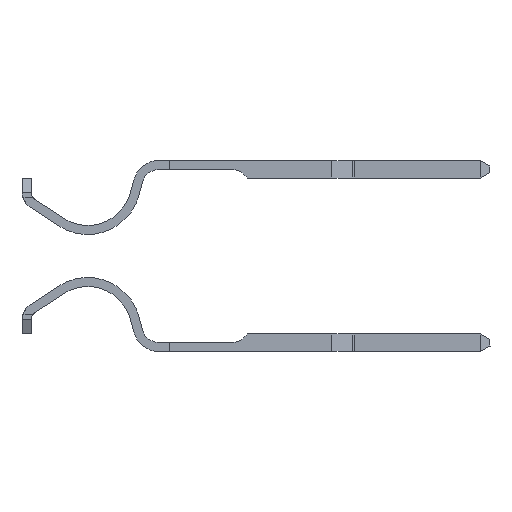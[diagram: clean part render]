
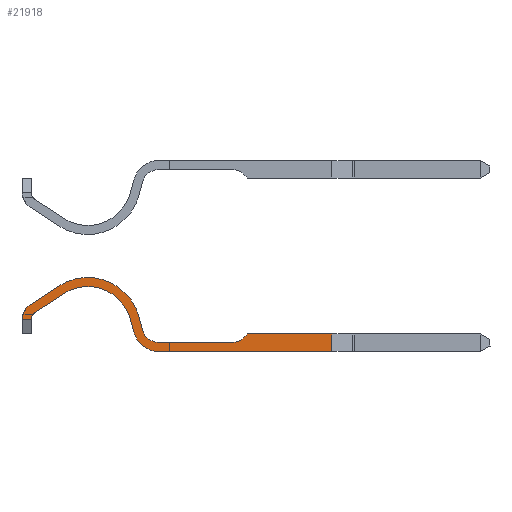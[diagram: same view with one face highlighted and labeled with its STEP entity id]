
A CAD part, left-side view. The second image highlights one B-rep face of the part: STEP entity #21918.
In plain terms, the highlighted face is planar.
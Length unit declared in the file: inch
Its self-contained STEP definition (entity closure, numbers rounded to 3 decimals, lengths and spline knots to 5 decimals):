
#345 = DIRECTION ( 'NONE',  ( 0., 0., -1. ) ) ;
#789 = DIRECTION ( 'NONE',  ( 0.836, 0.549, 0. ) ) ;
#810 = DIRECTION ( 'NONE',  ( 1., 0., 0. ) ) ;
#1173 = CARTESIAN_POINT ( 'NONE',  ( 0.43721, 0.04723, 0.025 ) ) ;
#1395 = DIRECTION ( 'NONE',  ( 1., 0., 0. ) ) ;
#1508 = VERTEX_POINT ( 'NONE', #23892 ) ;
#1675 = CARTESIAN_POINT ( 'NONE',  ( 0.18604, 0.10646, 0.025 ) ) ;
#1725 = VERTEX_POINT ( 'NONE', #7001 ) ;
#1872 = ORIENTED_EDGE ( 'NONE', *, *, #14459, .T. ) ;
#1982 = EDGE_CURVE ( 'NONE', #22254, #22426, #15676, .T. ) ;
#2128 = ORIENTED_EDGE ( 'NONE', *, *, #11549, .T. ) ;
#2558 = PLANE ( 'NONE',  #15448 ) ;
#2674 = CARTESIAN_POINT ( 'NONE',  ( 0.33, 0.0255, 0.025 ) ) ;
#2979 = ORIENTED_EDGE ( 'NONE', *, *, #1982, .T. ) ;
#3104 = CARTESIAN_POINT ( 'NONE',  ( 0.28917, 0.05955, 0.025 ) ) ;
#3242 = CARTESIAN_POINT ( 'NONE',  ( 0.30169, 0.06304, 0.025 ) ) ;
#3529 = DIRECTION ( 'NONE',  ( 0.836, 0.549, 0. ) ) ;
#3743 = ORIENTED_EDGE ( 'NONE', *, *, #25548, .T. ) ;
#3949 = CARTESIAN_POINT ( 'NONE',  ( 0.13322, 0.058, 0.025 ) ) ;
#4133 = CARTESIAN_POINT ( 'NONE',  ( 0.29484, 0.0392, 0.025 ) ) ;
#4280 = DIRECTION ( 'NONE',  ( 0., 0., 1. ) ) ;
#4358 = EDGE_CURVE ( 'NONE', #13284, #9220, #6090, .T. ) ;
#4414 = CIRCLE ( 'NONE', #4986, 0.0135 ) ;
#4643 = EDGE_CURVE ( 'NONE', #25637, #8201, #14313, .T. ) ;
#4644 = AXIS2_PLACEMENT_3D ( 'NONE', #1173, #345, #810 ) ;
#4709 = CARTESIAN_POINT ( 'NONE',  ( 0.095, 0.025, 0.025 ) ) ;
#4986 = AXIS2_PLACEMENT_3D ( 'NONE', #21334, #8874, #23396 ) ;
#5093 = EDGE_CURVE ( 'NONE', #15877, #24481, #4414, .T. ) ;
#5135 = CARTESIAN_POINT ( 'NONE',  ( 0.14622, 0.058, 0.025 ) ) ;
#5580 = ORIENTED_EDGE ( 'NONE', *, *, #9966, .F. ) ;
#6068 = ORIENTED_EDGE ( 'NONE', *, *, #4643, .F. ) ;
#6090 = CIRCLE ( 'NONE', #4644, 0.02173 ) ;
#6138 = DIRECTION ( 'NONE',  ( 0., -1., 0. ) ) ;
#6139 = CARTESIAN_POINT ( 'NONE',  ( 0.33, 0.049, 0.025 ) ) ;
#6145 = LINE ( 'NONE', #11100, #22109 ) ;
#6302 = CARTESIAN_POINT ( 'NONE',  ( 0.30736, 0.04269, 0.025 ) ) ;
#6824 = DIRECTION ( 'NONE',  ( 0., 0., -1. ) ) ;
#6916 = VERTEX_POINT ( 'NONE', #14846 ) ;
#7001 = CARTESIAN_POINT ( 'NONE',  ( 0.58021, 0.0375, 0.025 ) ) ;
#7007 = CARTESIAN_POINT ( 'NONE',  ( 0.228, 0.0425, 0.025 ) ) ;
#7172 = VERTEX_POINT ( 'NONE', #7192 ) ;
#7192 = CARTESIAN_POINT ( 'NONE',  ( 0.19317, 0.09559, 0.025 ) ) ;
#7235 = CARTESIAN_POINT ( 'NONE',  ( 0.15231, 0.06879, 0.025 ) ) ;
#7249 = ORIENTED_EDGE ( 'NONE', *, *, #10610, .F. ) ;
#7564 = DIRECTION ( 'NONE',  ( -1., 0., 0. ) ) ;
#7816 = CARTESIAN_POINT ( 'NONE',  ( 0.28917, 0.05955, 0.025 ) ) ;
#7854 = AXIS2_PLACEMENT_3D ( 'NONE', #9623, #24112, #11756 ) ;
#8201 = VERTEX_POINT ( 'NONE', #10820 ) ;
#8260 = DIRECTION ( 'NONE',  ( 1., 0., 0. ) ) ;
#8293 = VERTEX_POINT ( 'NONE', #2674 ) ;
#8311 = ORIENTED_EDGE ( 'NONE', *, *, #5093, .T. ) ;
#8508 = VECTOR ( 'NONE', #3529, 39.37008 ) ;
#8747 = ORIENTED_EDGE ( 'NONE', *, *, #10724, .T. ) ;
#8874 = DIRECTION ( 'NONE',  ( 0., 0., -1. ) ) ;
#8889 = ORIENTED_EDGE ( 'NONE', *, *, #27008, .T. ) ;
#9102 = ORIENTED_EDGE ( 'NONE', *, *, #16155, .F. ) ;
#9114 = DIRECTION ( 'NONE',  ( -1., 0., 0. ) ) ;
#9220 = VERTEX_POINT ( 'NONE', #9662 ) ;
#9623 = CARTESIAN_POINT ( 'NONE',  ( 0.15971, 0.0575, 0.025 ) ) ;
#9662 = CARTESIAN_POINT ( 'NONE',  ( 0.43721, 0.0255, 0.025 ) ) ;
#9685 = EDGE_LOOP ( 'NONE', ( #10353, #8747, #8311, #8889, #10164, #2979, #10428, #1872, #25355, #2128, #3743, #12183, #16659, #9102, #7249, #6068, #5580 ) ) ;
#9966 = EDGE_CURVE ( 'NONE', #12406, #25637, #19583, .T. ) ;
#10072 = LINE ( 'NONE', #25475, #25895 ) ;
#10164 = ORIENTED_EDGE ( 'NONE', *, *, #15193, .T. ) ;
#10212 = EDGE_CURVE ( 'NONE', #22426, #6916, #24711, .T. ) ;
#10353 = ORIENTED_EDGE ( 'NONE', *, *, #19406, .F. ) ;
#10428 = ORIENTED_EDGE ( 'NONE', *, *, #10212, .T. ) ;
#10610 = EDGE_CURVE ( 'NONE', #8201, #13938, #21800, .T. ) ;
#10724 = EDGE_CURVE ( 'NONE', #24245, #15877, #13078, .T. ) ;
#10820 = CARTESIAN_POINT ( 'NONE',  ( 0.30169, 0.06304, 0.025 ) ) ;
#10937 = DIRECTION ( 'NONE',  ( 1., 0., 0. ) ) ;
#11100 = CARTESIAN_POINT ( 'NONE',  ( 0.33, 0.0125, 0.025 ) ) ;
#11393 = CIRCLE ( 'NONE', #18821, 0.0635 ) ;
#11549 = EDGE_CURVE ( 'NONE', #1725, #1508, #10072, .T. ) ;
#11756 = DIRECTION ( 'NONE',  ( -1., 0., 0. ) ) ;
#12002 = CARTESIAN_POINT ( 'NONE',  ( 0.45821, 0.0375, 0.025 ) ) ;
#12054 = VECTOR ( 'NONE', #6138, 39.37008 ) ;
#12183 = ORIENTED_EDGE ( 'NONE', *, *, #4358, .T. ) ;
#12406 = VERTEX_POINT ( 'NONE', #18382 ) ;
#12574 = LINE ( 'NONE', #23333, #18097 ) ;
#13078 = LINE ( 'NONE', #20290, #17952 ) ;
#13147 = DIRECTION ( 'NONE',  ( -1., 0., 0. ) ) ;
#13284 = VERTEX_POINT ( 'NONE', #20920 ) ;
#13657 = DIRECTION ( 'NONE',  ( 0.268, -0.963, 0. ) ) ;
#13938 = VERTEX_POINT ( 'NONE', #6302 ) ;
#14313 = CIRCLE ( 'NONE', #21411, 0.0765 ) ;
#14459 = EDGE_CURVE ( 'NONE', #6916, #21876, #6145, .T. ) ;
#14846 = CARTESIAN_POINT ( 'NONE',  ( 0.33, 0.0125, 0.025 ) ) ;
#14996 = CARTESIAN_POINT ( 'NONE',  ( 0.58021, 0.0125, 0.025 ) ) ;
#15193 = EDGE_CURVE ( 'NONE', #7172, #22254, #11393, .T. ) ;
#15290 = FACE_OUTER_BOUND ( 'NONE', #9685, .T. ) ;
#15448 = AXIS2_PLACEMENT_3D ( 'NONE', #4709, #6824, #21393 ) ;
#15465 = LINE ( 'NONE', #7235, #25746 ) ;
#15659 = VECTOR ( 'NONE', #15803, 39.37008 ) ;
#15676 = LINE ( 'NONE', #3104, #26595 ) ;
#15803 = DIRECTION ( 'NONE',  ( 0.268, -0.963, 0. ) ) ;
#15877 = VERTEX_POINT ( 'NONE', #5135 ) ;
#16155 = EDGE_CURVE ( 'NONE', #13938, #8293, #24582, .T. ) ;
#16659 = ORIENTED_EDGE ( 'NONE', *, *, #26438, .F. ) ;
#16854 = CARTESIAN_POINT ( 'NONE',  ( 0.33, 0.049, 0.025 ) ) ;
#17156 = CARTESIAN_POINT ( 'NONE',  ( 0.15231, 0.06879, 0.025 ) ) ;
#17952 = VECTOR ( 'NONE', #1395, 39.37008 ) ;
#18097 = VECTOR ( 'NONE', #10937, 39.37008 ) ;
#18150 = VECTOR ( 'NONE', #24341, 39.37008 ) ;
#18382 = CARTESIAN_POINT ( 'NONE',  ( 0.14518, 0.07966, 0.025 ) ) ;
#18821 = AXIS2_PLACEMENT_3D ( 'NONE', #7007, #21584, #9114 ) ;
#18896 = DIRECTION ( 'NONE',  ( 1., 0., 0. ) ) ;
#19406 = EDGE_CURVE ( 'NONE', #24245, #12406, #21526, .T. ) ;
#19583 = LINE ( 'NONE', #26327, #8508 ) ;
#20024 = AXIS2_PLACEMENT_3D ( 'NONE', #6139, #20720, #8260 ) ;
#20127 = CARTESIAN_POINT ( 'NONE',  ( 0.228, 0.0425, 0.025 ) ) ;
#20290 = CARTESIAN_POINT ( 'NONE',  ( 0.14621, 0.058, 0.025 ) ) ;
#20719 = CARTESIAN_POINT ( 'NONE',  ( 0.58021, 0.0375, 0.025 ) ) ;
#20720 = DIRECTION ( 'NONE',  ( 0., 0., 1. ) ) ;
#20920 = CARTESIAN_POINT ( 'NONE',  ( 0.45258, 0.03186, 0.025 ) ) ;
#21334 = CARTESIAN_POINT ( 'NONE',  ( 0.15971, 0.0575, 0.025 ) ) ;
#21393 = DIRECTION ( 'NONE',  ( -1., 0., 0. ) ) ;
#21411 = AXIS2_PLACEMENT_3D ( 'NONE', #20127, #22987, #7564 ) ;
#21526 = CIRCLE ( 'NONE', #7854, 0.0265 ) ;
#21584 = DIRECTION ( 'NONE',  ( 0., 0., -1. ) ) ;
#21800 = LINE ( 'NONE', #3242, #15659 ) ;
#21876 = VERTEX_POINT ( 'NONE', #14996 ) ;
#21918 = ADVANCED_FACE ( 'NONE', ( #15290 ), #2558, .F. ) ;
#22109 = VECTOR ( 'NONE', #23506, 39.37008 ) ;
#22254 = VERTEX_POINT ( 'NONE', #7816 ) ;
#22391 = LINE ( 'NONE', #20719, #12054 ) ;
#22426 = VERTEX_POINT ( 'NONE', #4133 ) ;
#22987 = DIRECTION ( 'NONE',  ( 0., 0., -1. ) ) ;
#23333 = CARTESIAN_POINT ( 'NONE',  ( 0.33, 0.0255, 0.025 ) ) ;
#23396 = DIRECTION ( 'NONE',  ( -1., 0., 0. ) ) ;
#23506 = DIRECTION ( 'NONE',  ( 1., 0., 0. ) ) ;
#23602 = LINE ( 'NONE', #12002, #18150 ) ;
#23892 = CARTESIAN_POINT ( 'NONE',  ( 0.45821, 0.0375, 0.025 ) ) ;
#24112 = DIRECTION ( 'NONE',  ( 0., 0., -1. ) ) ;
#24245 = VERTEX_POINT ( 'NONE', #3949 ) ;
#24298 = EDGE_CURVE ( 'NONE', #1725, #21876, #22391, .T. ) ;
#24341 = DIRECTION ( 'NONE',  ( -0.707, -0.707, 0. ) ) ;
#24481 = VERTEX_POINT ( 'NONE', #17156 ) ;
#24582 = CIRCLE ( 'NONE', #20024, 0.0235 ) ;
#24711 = CIRCLE ( 'NONE', #25579, 0.0365 ) ;
#25355 = ORIENTED_EDGE ( 'NONE', *, *, #24298, .F. ) ;
#25475 = CARTESIAN_POINT ( 'NONE',  ( 0.45821, 0.0375, 0.025 ) ) ;
#25548 = EDGE_CURVE ( 'NONE', #1508, #13284, #23602, .T. ) ;
#25579 = AXIS2_PLACEMENT_3D ( 'NONE', #16854, #4280, #18896 ) ;
#25637 = VERTEX_POINT ( 'NONE', #1675 ) ;
#25746 = VECTOR ( 'NONE', #789, 39.37008 ) ;
#25895 = VECTOR ( 'NONE', #13147, 39.37008 ) ;
#26327 = CARTESIAN_POINT ( 'NONE',  ( 0.14518, 0.07966, 0.025 ) ) ;
#26438 = EDGE_CURVE ( 'NONE', #8293, #9220, #12574, .T. ) ;
#26595 = VECTOR ( 'NONE', #13657, 39.37008 ) ;
#27008 = EDGE_CURVE ( 'NONE', #24481, #7172, #15465, .T. ) ;
